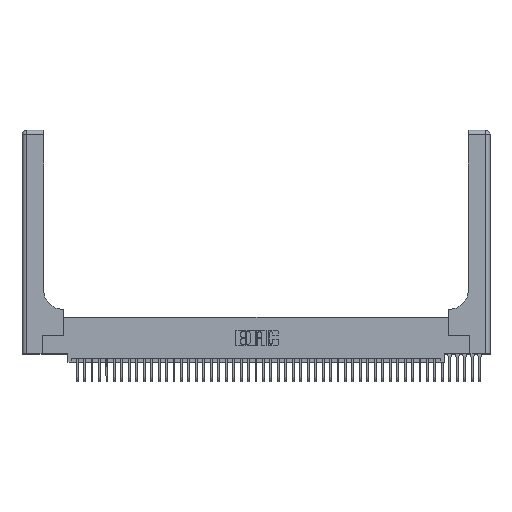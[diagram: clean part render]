
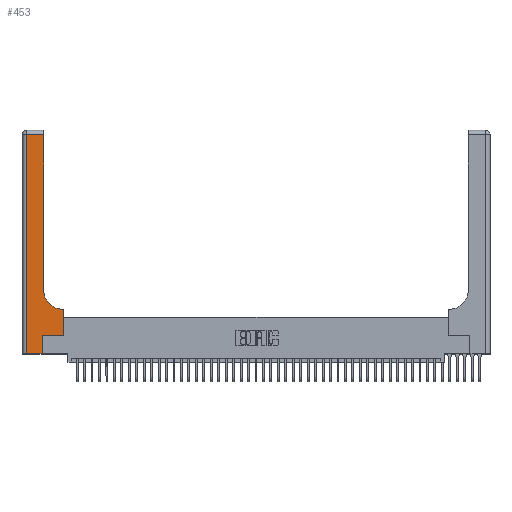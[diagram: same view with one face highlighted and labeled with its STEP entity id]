
A CAD part, top view. The second image highlights one B-rep face of the part: STEP entity #453.
In plain terms, the highlighted planar face has unit normal (0, 0, 1).
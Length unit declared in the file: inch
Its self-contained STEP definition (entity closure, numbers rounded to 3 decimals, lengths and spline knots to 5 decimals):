
#453 = ADVANCED_FACE ( 'NONE', ( #24130 ), #39617, .F. ) ;
#1102 = LINE ( 'NONE', #15237, #33309 ) ;
#1526 = VERTEX_POINT ( 'NONE', #18657 ) ;
#1627 = CARTESIAN_POINT ( 'NONE',  ( 0.06, 2.94, 0.37 ) ) ;
#1801 = ORIENTED_EDGE ( 'NONE', *, *, #28510, .T. ) ;
#2747 = VECTOR ( 'NONE', #25808, 39.37008 ) ;
#4397 = EDGE_CURVE ( 'NONE', #27078, #5691, #19419, .T. ) ;
#4460 = DIRECTION ( 'NONE',  ( -1., 0., 0. ) ) ;
#4859 = VECTOR ( 'NONE', #34246, 39.37008 ) ;
#5441 = ORIENTED_EDGE ( 'NONE', *, *, #37728, .T. ) ;
#5691 = VERTEX_POINT ( 'NONE', #37731 ) ;
#6221 = CARTESIAN_POINT ( 'NONE',  ( 0.5585, 0.25, 0.37 ) ) ;
#6477 = CARTESIAN_POINT ( 'NONE',  ( 0.2915, 3., 0.37 ) ) ;
#7426 = CARTESIAN_POINT ( 'NONE',  ( 0.5585, 0.6, 0.37 ) ) ;
#7499 = VECTOR ( 'NONE', #15608, 39.37008 ) ;
#8376 = EDGE_CURVE ( 'NONE', #36257, #26366, #10361, .T. ) ;
#9967 = CIRCLE ( 'NONE', #18514, 0.25 ) ;
#10361 = LINE ( 'NONE', #6477, #2747 ) ;
#10748 = CARTESIAN_POINT ( 'NONE',  ( 0.2915, 2.94, 0.37 ) ) ;
#10860 = VECTOR ( 'NONE', #31125, 39.37008 ) ;
#11883 = DIRECTION ( 'NONE',  ( 0., 0., -1. ) ) ;
#12032 = ORIENTED_EDGE ( 'NONE', *, *, #8376, .T. ) ;
#13305 = AXIS2_PLACEMENT_3D ( 'NONE', #20576, #23835, #4460 ) ;
#13916 = VERTEX_POINT ( 'NONE', #7426 ) ;
#15041 = CARTESIAN_POINT ( 'NONE',  ( 0.269, 0.25, 0.37 ) ) ;
#15237 = CARTESIAN_POINT ( 'NONE',  ( 0.269, 0., 0.37 ) ) ;
#15608 = DIRECTION ( 'NONE',  ( 0., 1., 0. ) ) ;
#17599 = LINE ( 'NONE', #26503, #35595 ) ;
#17941 = EDGE_CURVE ( 'NONE', #22936, #13916, #41466, .T. ) ;
#18514 = AXIS2_PLACEMENT_3D ( 'NONE', #31142, #11883, #34304 ) ;
#18609 = CARTESIAN_POINT ( 'NONE',  ( 0., 2.94, 0.37 ) ) ;
#18657 = CARTESIAN_POINT ( 'NONE',  ( 0.269, 0.25, 0.37 ) ) ;
#19068 = LINE ( 'NONE', #18609, #35042 ) ;
#19072 = ORIENTED_EDGE ( 'NONE', *, *, #4397, .T. ) ;
#19238 = CARTESIAN_POINT ( 'NONE',  ( 0.269, 0., 0.37 ) ) ;
#19419 = LINE ( 'NONE', #34287, #10860 ) ;
#19781 = CARTESIAN_POINT ( 'NONE',  ( 0., 0., 0.37 ) ) ;
#20576 = CARTESIAN_POINT ( 'NONE',  ( 0., 3., 0.37 ) ) ;
#20830 = ORIENTED_EDGE ( 'NONE', *, *, #17941, .T. ) ;
#21587 = CARTESIAN_POINT ( 'NONE',  ( 0.5415, 0.6, 0.37 ) ) ;
#21636 = VERTEX_POINT ( 'NONE', #21587 ) ;
#22936 = VERTEX_POINT ( 'NONE', #6221 ) ;
#23075 = DIRECTION ( 'NONE',  ( 1., 0., 0. ) ) ;
#23811 = CARTESIAN_POINT ( 'NONE',  ( 0.2915, 0.85, 0.37 ) ) ;
#23835 = DIRECTION ( 'NONE',  ( 0., 0., -1. ) ) ;
#24130 = FACE_OUTER_BOUND ( 'NONE', #36653, .T. ) ;
#24358 = ORIENTED_EDGE ( 'NONE', *, *, #32713, .T. ) ;
#25808 = DIRECTION ( 'NONE',  ( 0., 1., 0. ) ) ;
#26366 = VERTEX_POINT ( 'NONE', #10748 ) ;
#26503 = CARTESIAN_POINT ( 'NONE',  ( 0.2915, 0.6, 0.37 ) ) ;
#27078 = VERTEX_POINT ( 'NONE', #1627 ) ;
#28510 = EDGE_CURVE ( 'NONE', #26366, #27078, #19068, .T. ) ;
#28766 = ORIENTED_EDGE ( 'NONE', *, *, #38585, .T. ) ;
#29331 = EDGE_CURVE ( 'NONE', #1526, #22936, #31555, .T. ) ;
#29693 = DIRECTION ( 'NONE',  ( -1., 0., 0. ) ) ;
#31125 = DIRECTION ( 'NONE',  ( 0., -1., 0. ) ) ;
#31142 = CARTESIAN_POINT ( 'NONE',  ( 0.5415, 0.85, 0.37 ) ) ;
#31555 = LINE ( 'NONE', #15041, #4859 ) ;
#32713 = EDGE_CURVE ( 'NONE', #34173, #1526, #1102, .T. ) ;
#33309 = VECTOR ( 'NONE', #37596, 39.37008 ) ;
#33864 = VECTOR ( 'NONE', #23075, 39.37008 ) ;
#34173 = VERTEX_POINT ( 'NONE', #19238 ) ;
#34246 = DIRECTION ( 'NONE',  ( 1., 0., 0. ) ) ;
#34287 = CARTESIAN_POINT ( 'NONE',  ( 0.06, 3., 0.37 ) ) ;
#34304 = DIRECTION ( 'NONE',  ( 1., 0., 0. ) ) ;
#34538 = DIRECTION ( 'NONE',  ( -1., 0., 0. ) ) ;
#34821 = LINE ( 'NONE', #19781, #33864 ) ;
#34846 = EDGE_CURVE ( 'NONE', #5691, #34173, #34821, .T. ) ;
#35042 = VECTOR ( 'NONE', #34538, 39.37008 ) ;
#35595 = VECTOR ( 'NONE', #29693, 39.37008 ) ;
#36257 = VERTEX_POINT ( 'NONE', #23811 ) ;
#36653 = EDGE_LOOP ( 'NONE', ( #12032, #1801, #19072, #38421, #24358, #40788, #20830, #5441, #28766 ) ) ;
#37596 = DIRECTION ( 'NONE',  ( 0., 1., 0. ) ) ;
#37728 = EDGE_CURVE ( 'NONE', #13916, #21636, #17599, .T. ) ;
#37731 = CARTESIAN_POINT ( 'NONE',  ( 0.06, 0., 0.37 ) ) ;
#38421 = ORIENTED_EDGE ( 'NONE', *, *, #34846, .T. ) ;
#38585 = EDGE_CURVE ( 'NONE', #21636, #36257, #9967, .T. ) ;
#39617 = PLANE ( 'NONE',  #13305 ) ;
#40788 = ORIENTED_EDGE ( 'NONE', *, *, #29331, .T. ) ;
#41116 = CARTESIAN_POINT ( 'NONE',  ( 0.5585, 0.25, 0.37 ) ) ;
#41466 = LINE ( 'NONE', #41116, #7499 ) ;
